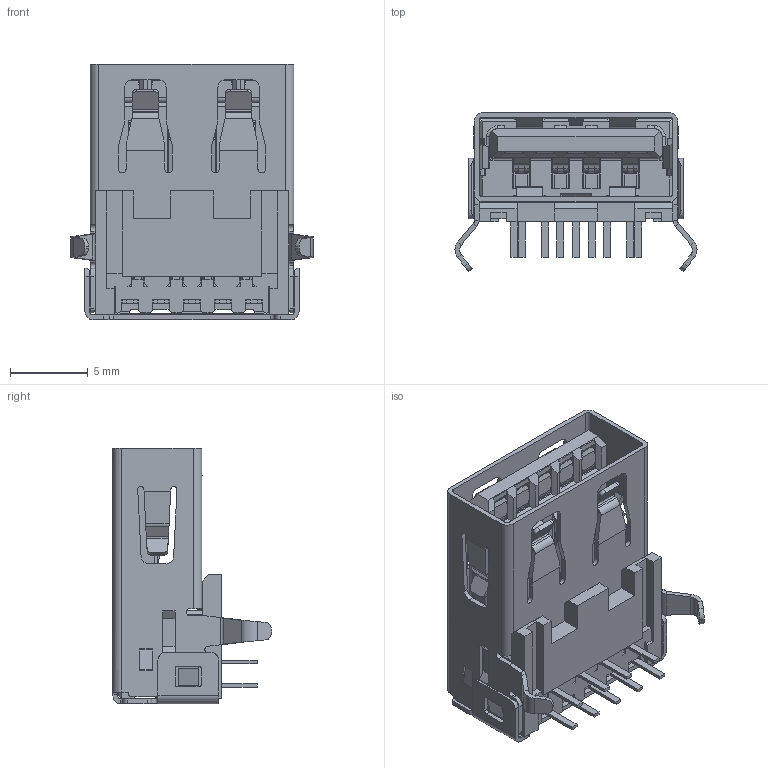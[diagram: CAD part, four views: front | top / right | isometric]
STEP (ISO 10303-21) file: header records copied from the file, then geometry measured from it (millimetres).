
FILE_DESCRIPTION (( 'STEP AP214' ), '1' );
FILE_NAME ('690B109-223-222.STEP', '2021-01-14T17:30:02', ( '' ), ( '' ), 'SwSTEP 2.0', 'SolidWorks 2020', '' );
FILE_SCHEMA (( 'AUTOMOTIVE_DESIGN' ));
Length unit declared in the file: millimetre
Products named in the file (4): Shell 690B109-X23-222; Insulator 690B109-X23-222; Contacts 690B109-X23-222; 690B109-223-222
Assembly tree (3 placements, depth 2):
  690B109-223-222
    Insulator 690B109-X23-222
    Contacts 690B109-X23-222
    Shell 690B109-X23-222
Bounding box: 15.6 x 10.26 x 16.45 mm (x, y, z)
Volume: 674.5 mm3; surface area: 3023.6 mm2
Topology: 11 solids, 11 shells, 2226 faces, 6503 edges, 4231 vertices
Faces by surface type: plane 1535, cylinder 553, bspline 130, torus 8
Entity records: 76249 total; most frequent: CARTESIAN_POINT 17415, ORIENTED_EDGE 13006, DIRECTION 11345, EDGE_CURVE 6503, LINE 5103, VECTOR 5103, VERTEX_POINT 4231, AXIS2_PLACEMENT_3D 3121
